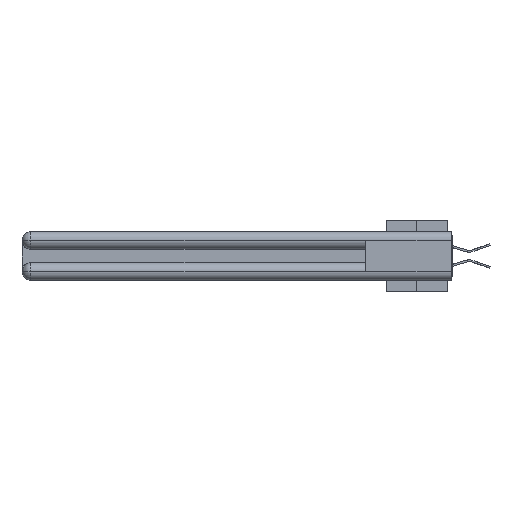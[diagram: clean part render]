
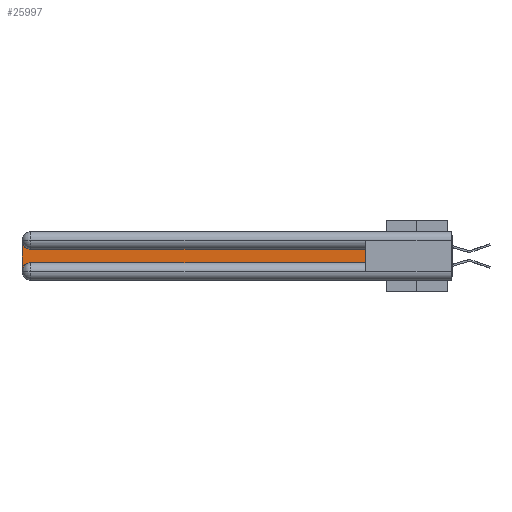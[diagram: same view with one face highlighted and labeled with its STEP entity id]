
A CAD part, left-side view. The second image highlights one B-rep face of the part: STEP entity #25997.
In plain terms, the highlighted planar face has unit normal (-1, 0, 0).
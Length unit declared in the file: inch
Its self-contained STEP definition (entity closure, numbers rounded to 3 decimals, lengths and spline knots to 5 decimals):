
#1605 = ORIENTED_EDGE ( 'NONE', *, *, #33749, .T. ) ;
#2723 = CIRCLE ( 'NONE', #38086, 0.06 ) ;
#3207 = PLANE ( 'NONE',  #42552 ) ;
#3259 = CARTESIAN_POINT ( 'NONE',  ( 0.075, 3., -0.2775 ) ) ;
#3380 = VERTEX_POINT ( 'NONE', #22509 ) ;
#3563 = CARTESIAN_POINT ( 'NONE',  ( 0.075, 3., -0.0625 ) ) ;
#3641 = LINE ( 'NONE', #18904, #16825 ) ;
#4157 = DIRECTION ( 'NONE',  ( 0., 0., 1. ) ) ;
#5312 = EDGE_CURVE ( 'NONE', #40675, #32751, #22321, .T. ) ;
#6057 = EDGE_CURVE ( 'NONE', #32374, #3380, #13265, .T. ) ;
#6319 = CARTESIAN_POINT ( 'NONE',  ( 0.075, 2.94, -0.2775 ) ) ;
#6828 = DIRECTION ( 'NONE',  ( 0., 0., -1. ) ) ;
#7336 = EDGE_CURVE ( 'NONE', #32751, #14574, #21524, .T. ) ;
#10454 = CARTESIAN_POINT ( 'NONE',  ( 0.075, 3., -0.2175 ) ) ;
#11583 = ORIENTED_EDGE ( 'NONE', *, *, #5312, .T. ) ;
#13265 = LINE ( 'NONE', #35275, #38992 ) ;
#14574 = VERTEX_POINT ( 'NONE', #38996 ) ;
#15489 = CARTESIAN_POINT ( 'NONE',  ( 0.075, 0.6, -0.2175 ) ) ;
#16825 = VECTOR ( 'NONE', #4157, 39.37008 ) ;
#17443 = EDGE_LOOP ( 'NONE', ( #26141, #21819, #33698, #11583, #29853, #1605 ) ) ;
#18904 = CARTESIAN_POINT ( 'NONE',  ( 0.075, 0.6, -0.2175 ) ) ;
#19693 = EDGE_CURVE ( 'NONE', #3380, #46528, #2723, .T. ) ;
#19947 = CARTESIAN_POINT ( 'NONE',  ( 0.075, 0.6, -0.1225 ) ) ;
#21364 = CARTESIAN_POINT ( 'NONE',  ( 0.075, 2.94, -0.2175 ) ) ;
#21524 = LINE ( 'NONE', #15489, #47305 ) ;
#21819 = ORIENTED_EDGE ( 'NONE', *, *, #19693, .T. ) ;
#22250 = DIRECTION ( 'NONE',  ( 1., 0., 0. ) ) ;
#22321 = CIRCLE ( 'NONE', #24536, 0.06 ) ;
#22509 = CARTESIAN_POINT ( 'NONE',  ( 0.075, 2.94, -0.1225 ) ) ;
#24536 = AXIS2_PLACEMENT_3D ( 'NONE', #6319, #44843, #33089 ) ;
#25844 = VECTOR ( 'NONE', #45282, 39.37008 ) ;
#25997 = ADVANCED_FACE ( 'NONE', ( #32987 ), #3207, .F. ) ;
#26141 = ORIENTED_EDGE ( 'NONE', *, *, #6057, .T. ) ;
#29853 = ORIENTED_EDGE ( 'NONE', *, *, #7336, .T. ) ;
#30847 = DIRECTION ( 'NONE',  ( 0., -1., 0. ) ) ;
#32374 = VERTEX_POINT ( 'NONE', #19947 ) ;
#32751 = VERTEX_POINT ( 'NONE', #21364 ) ;
#32987 = FACE_OUTER_BOUND ( 'NONE', #17443, .T. ) ;
#33089 = DIRECTION ( 'NONE',  ( 0., 0., -1. ) ) ;
#33698 = ORIENTED_EDGE ( 'NONE', *, *, #42235, .T. ) ;
#33749 = EDGE_CURVE ( 'NONE', #14574, #32374, #3641, .T. ) ;
#33844 = DIRECTION ( 'NONE',  ( 1., 0., 0. ) ) ;
#35275 = CARTESIAN_POINT ( 'NONE',  ( 0.075, 0.6, -0.1225 ) ) ;
#35432 = DIRECTION ( 'NONE',  ( 0., 1., 0. ) ) ;
#36025 = LINE ( 'NONE', #10454, #25844 ) ;
#37457 = CARTESIAN_POINT ( 'NONE',  ( 0.075, 2.94, -0.0625 ) ) ;
#38086 = AXIS2_PLACEMENT_3D ( 'NONE', #37457, #22250, #6828 ) ;
#38992 = VECTOR ( 'NONE', #35432, 39.37008 ) ;
#38996 = CARTESIAN_POINT ( 'NONE',  ( 0.075, 0.6, -0.2175 ) ) ;
#40675 = VERTEX_POINT ( 'NONE', #3259 ) ;
#41570 = CARTESIAN_POINT ( 'NONE',  ( 0.075, 3., -0.1225 ) ) ;
#42235 = EDGE_CURVE ( 'NONE', #46528, #40675, #36025, .T. ) ;
#42552 = AXIS2_PLACEMENT_3D ( 'NONE', #41570, #33844, #46800 ) ;
#44843 = DIRECTION ( 'NONE',  ( 1., 0., 0. ) ) ;
#45282 = DIRECTION ( 'NONE',  ( 0., 0., -1. ) ) ;
#46528 = VERTEX_POINT ( 'NONE', #3563 ) ;
#46800 = DIRECTION ( 'NONE',  ( 0., 0., -1. ) ) ;
#47305 = VECTOR ( 'NONE', #30847, 39.37008 ) ;
